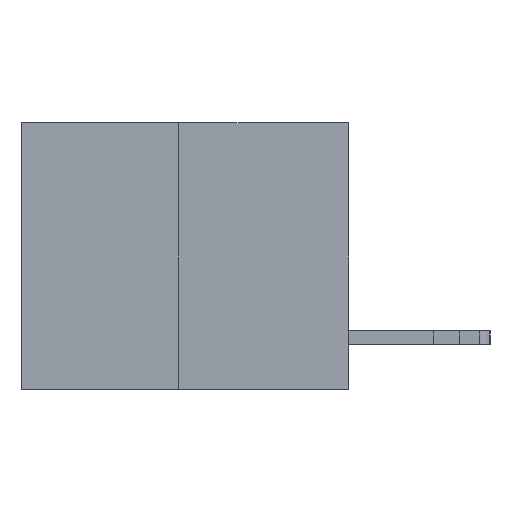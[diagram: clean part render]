
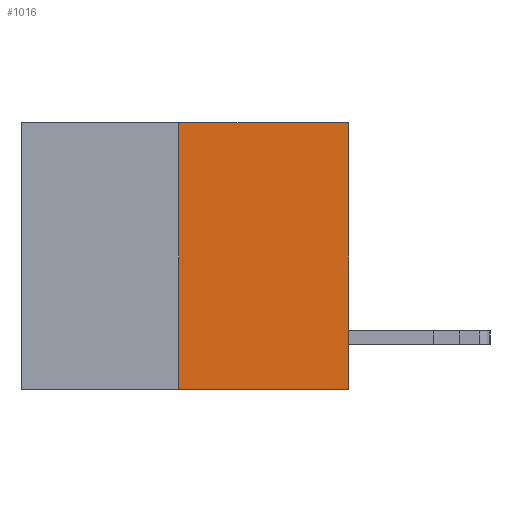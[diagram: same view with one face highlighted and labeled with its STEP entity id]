
A CAD part, left-side view. The second image highlights one B-rep face of the part: STEP entity #1016.
In plain terms, the highlighted planar face has unit normal (-1, 0, 0).
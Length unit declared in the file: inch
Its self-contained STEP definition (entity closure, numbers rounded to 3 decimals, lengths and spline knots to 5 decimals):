
#144 = DIRECTION ( 'NONE',  ( 0., -1., 0. ) ) ;
#504 = CARTESIAN_POINT ( 'NONE',  ( 0., 0., 0. ) ) ;
#545 = DIRECTION ( 'NONE',  ( 0., 0., 1. ) ) ;
#733 = LINE ( 'NONE', #12993, #11824 ) ;
#911 = EDGE_LOOP ( 'NONE', ( #11859, #12707, #1710, #4472 ) ) ;
#1016 = ADVANCED_FACE ( 'NONE', ( #7338 ), #11389, .F. ) ;
#1659 = AXIS2_PLACEMENT_3D ( 'NONE', #11470, #7193, #5296 ) ;
#1710 = ORIENTED_EDGE ( 'NONE', *, *, #5922, .T. ) ;
#2321 = VECTOR ( 'NONE', #11704, 39.37008 ) ;
#3109 = VECTOR ( 'NONE', #545, 39.37008 ) ;
#3123 = VERTEX_POINT ( 'NONE', #12916 ) ;
#3191 = CARTESIAN_POINT ( 'NONE',  ( 0., 0.6, -0.49 ) ) ;
#3856 = CARTESIAN_POINT ( 'NONE',  ( 0., 0.312, -0.49 ) ) ;
#4472 = ORIENTED_EDGE ( 'NONE', *, *, #4873, .F. ) ;
#4476 = CARTESIAN_POINT ( 'NONE',  ( 0., 0.312, -0.49 ) ) ;
#4511 = LINE ( 'NONE', #3191, #7587 ) ;
#4652 = DIRECTION ( 'NONE',  ( 0., -1., 0. ) ) ;
#4873 = EDGE_CURVE ( 'NONE', #3123, #9761, #733, .T. ) ;
#5296 = DIRECTION ( 'NONE',  ( 0., 0., -1. ) ) ;
#5360 = LINE ( 'NONE', #504, #3109 ) ;
#5389 = EDGE_CURVE ( 'NONE', #11054, #3123, #9236, .T. ) ;
#5922 = EDGE_CURVE ( 'NONE', #11330, #9761, #5360, .T. ) ;
#6066 = CARTESIAN_POINT ( 'NONE',  ( 0., 0., -0.49 ) ) ;
#7193 = DIRECTION ( 'NONE',  ( 1., 0., 0. ) ) ;
#7338 = FACE_OUTER_BOUND ( 'NONE', #911, .T. ) ;
#7587 = VECTOR ( 'NONE', #144, 39.37008 ) ;
#9236 = LINE ( 'NONE', #4476, #2321 ) ;
#9761 = VERTEX_POINT ( 'NONE', #11851 ) ;
#10036 = EDGE_CURVE ( 'NONE', #11054, #11330, #4511, .T. ) ;
#11054 = VERTEX_POINT ( 'NONE', #3856 ) ;
#11330 = VERTEX_POINT ( 'NONE', #6066 ) ;
#11389 = PLANE ( 'NONE',  #1659 ) ;
#11470 = CARTESIAN_POINT ( 'NONE',  ( 0., 0.6, 0. ) ) ;
#11704 = DIRECTION ( 'NONE',  ( 0., 0., 1. ) ) ;
#11824 = VECTOR ( 'NONE', #4652, 39.37008 ) ;
#11851 = CARTESIAN_POINT ( 'NONE',  ( 0., 0., 0. ) ) ;
#11859 = ORIENTED_EDGE ( 'NONE', *, *, #5389, .F. ) ;
#12707 = ORIENTED_EDGE ( 'NONE', *, *, #10036, .T. ) ;
#12916 = CARTESIAN_POINT ( 'NONE',  ( 0., 0.312, 0. ) ) ;
#12993 = CARTESIAN_POINT ( 'NONE',  ( 0., 0.6, 0. ) ) ;
